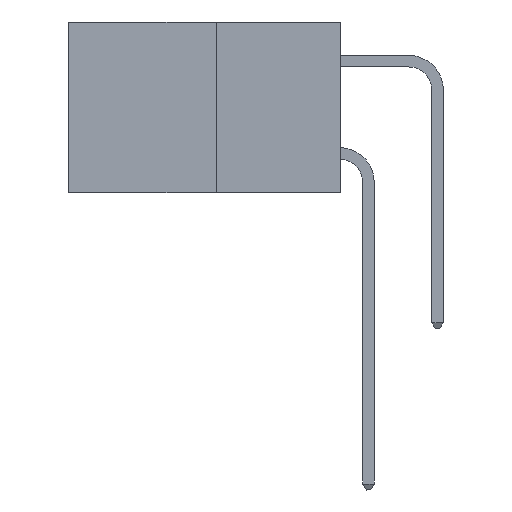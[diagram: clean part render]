
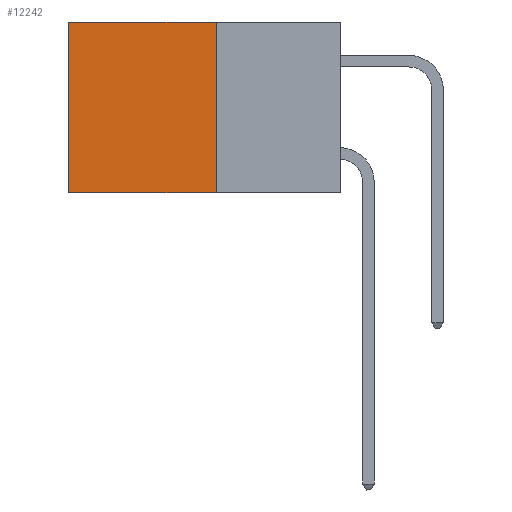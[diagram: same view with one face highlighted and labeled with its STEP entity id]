
A CAD part, left-side view. The second image highlights one B-rep face of the part: STEP entity #12242.
In plain terms, the highlighted planar face has unit normal (-1, 0, 0).
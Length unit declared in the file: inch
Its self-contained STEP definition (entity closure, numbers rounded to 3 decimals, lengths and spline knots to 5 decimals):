
#1431 = VERTEX_POINT ( 'NONE', #21962 ) ;
#2012 = VERTEX_POINT ( 'NONE', #4025 ) ;
#2289 = AXIS2_PLACEMENT_3D ( 'NONE', #14700, #3409, #16563 ) ;
#2596 = LINE ( 'NONE', #8555, #5809 ) ;
#2691 = LINE ( 'NONE', #19034, #12143 ) ;
#3409 = DIRECTION ( 'NONE',  ( 1., 0., 0. ) ) ;
#4025 = CARTESIAN_POINT ( 'NONE',  ( 0.277, 0.27, -0.37 ) ) ;
#4266 = ORIENTED_EDGE ( 'NONE', *, *, #19181, .T. ) ;
#4413 = FACE_OUTER_BOUND ( 'NONE', #18305, .T. ) ;
#5809 = VECTOR ( 'NONE', #23344, 39.37008 ) ;
#7334 = ORIENTED_EDGE ( 'NONE', *, *, #8065, .T. ) ;
#8065 = EDGE_CURVE ( 'NONE', #1431, #21077, #2596, .T. ) ;
#8555 = CARTESIAN_POINT ( 'NONE',  ( 0.277, 0.27, 0. ) ) ;
#8989 = VECTOR ( 'NONE', #10615, 39.37008 ) ;
#9373 = CARTESIAN_POINT ( 'NONE',  ( 0.277, 0.59, -0.37 ) ) ;
#9970 = ORIENTED_EDGE ( 'NONE', *, *, #18957, .F. ) ;
#10615 = DIRECTION ( 'NONE',  ( 0., 1., 0. ) ) ;
#11256 = DIRECTION ( 'NONE',  ( 0., 0., -1. ) ) ;
#11403 = CARTESIAN_POINT ( 'NONE',  ( 0.277, 0.59, -0.37 ) ) ;
#11673 = DIRECTION ( 'NONE',  ( 0., 0., -1. ) ) ;
#12143 = VECTOR ( 'NONE', #11673, 39.37008 ) ;
#12242 = ADVANCED_FACE ( 'NONE', ( #4413 ), #21982, .F. ) ;
#13665 = VECTOR ( 'NONE', #11256, 39.37008 ) ;
#14609 = EDGE_CURVE ( 'NONE', #1431, #2012, #2691, .T. ) ;
#14688 = CARTESIAN_POINT ( 'NONE',  ( 0.277, 0.59, 0. ) ) ;
#14700 = CARTESIAN_POINT ( 'NONE',  ( 0.277, 0.27, -0.37 ) ) ;
#16563 = DIRECTION ( 'NONE',  ( 0., 0., -1. ) ) ;
#17027 = ORIENTED_EDGE ( 'NONE', *, *, #14609, .F. ) ;
#17904 = VERTEX_POINT ( 'NONE', #11403 ) ;
#18305 = EDGE_LOOP ( 'NONE', ( #4266, #9970, #17027, #7334 ) ) ;
#18957 = EDGE_CURVE ( 'NONE', #2012, #17904, #23718, .T. ) ;
#19034 = CARTESIAN_POINT ( 'NONE',  ( 0.277, 0.27, -0.37 ) ) ;
#19181 = EDGE_CURVE ( 'NONE', #21077, #17904, #23395, .T. ) ;
#21077 = VERTEX_POINT ( 'NONE', #14688 ) ;
#21962 = CARTESIAN_POINT ( 'NONE',  ( 0.277, 0.27, 0. ) ) ;
#21982 = PLANE ( 'NONE',  #2289 ) ;
#23344 = DIRECTION ( 'NONE',  ( 0., 1., 0. ) ) ;
#23395 = LINE ( 'NONE', #9373, #13665 ) ;
#23519 = CARTESIAN_POINT ( 'NONE',  ( 0.277, 0.27, -0.37 ) ) ;
#23718 = LINE ( 'NONE', #23519, #8989 ) ;
